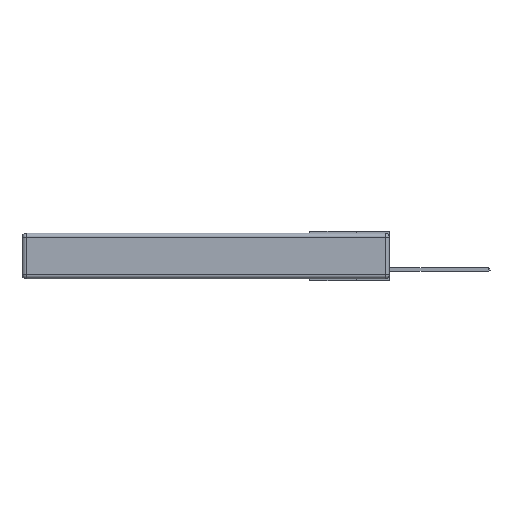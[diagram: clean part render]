
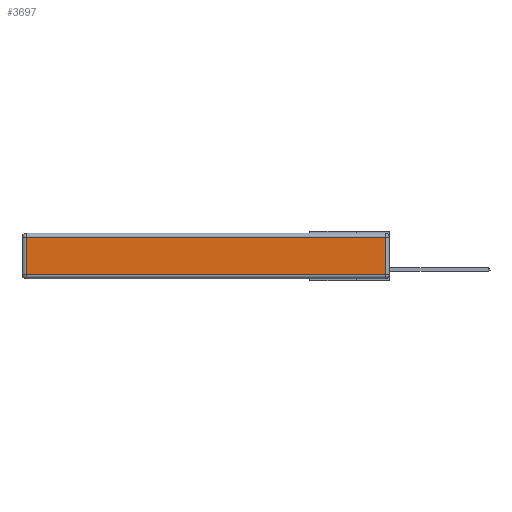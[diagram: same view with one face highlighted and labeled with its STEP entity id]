
A CAD part, left-side view. The second image highlights one B-rep face of the part: STEP entity #3697.
In plain terms, the highlighted planar face has unit normal (-1, 0, 0).
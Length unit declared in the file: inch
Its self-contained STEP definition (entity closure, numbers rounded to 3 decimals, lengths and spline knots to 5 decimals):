
#84 = VECTOR ( 'NONE', #12034, 39.37008 ) ;
#610 = PLANE ( 'NONE',  #6020 ) ;
#896 = VECTOR ( 'NONE', #3860, 39.37008 ) ;
#1994 = EDGE_LOOP ( 'NONE', ( #2185, #12031, #16019, #4994 ) ) ;
#2100 = CARTESIAN_POINT ( 'NONE',  ( 0., 0.03, -0.313 ) ) ;
#2173 = EDGE_CURVE ( 'NONE', #8842, #8181, #16119, .T. ) ;
#2185 = ORIENTED_EDGE ( 'NONE', *, *, #2173, .T. ) ;
#2301 = CARTESIAN_POINT ( 'NONE',  ( 0., 2.72, -0.03 ) ) ;
#2594 = CARTESIAN_POINT ( 'NONE',  ( 0., 0.03, -0.343 ) ) ;
#2646 = EDGE_CURVE ( 'NONE', #13889, #8842, #9479, .T. ) ;
#3697 = ADVANCED_FACE ( 'NONE', ( #5095 ), #610, .T. ) ;
#3860 = DIRECTION ( 'NONE',  ( 0., 0., 1. ) ) ;
#4325 = VERTEX_POINT ( 'NONE', #12150 ) ;
#4994 = ORIENTED_EDGE ( 'NONE', *, *, #2646, .T. ) ;
#5095 = FACE_OUTER_BOUND ( 'NONE', #1994, .T. ) ;
#6020 = AXIS2_PLACEMENT_3D ( 'NONE', #15780, #9581, #9794 ) ;
#6124 = VECTOR ( 'NONE', #11305, 39.37008 ) ;
#6652 = DIRECTION ( 'NONE',  ( 0., 1., 0. ) ) ;
#7256 = EDGE_CURVE ( 'NONE', #8181, #4325, #8352, .T. ) ;
#7280 = EDGE_CURVE ( 'NONE', #4325, #13889, #9692, .T. ) ;
#7716 = CARTESIAN_POINT ( 'NONE',  ( 0., 2.72, -0.313 ) ) ;
#8181 = VERTEX_POINT ( 'NONE', #2100 ) ;
#8352 = LINE ( 'NONE', #2594, #896 ) ;
#8842 = VERTEX_POINT ( 'NONE', #7716 ) ;
#9479 = LINE ( 'NONE', #14779, #6124 ) ;
#9581 = DIRECTION ( 'NONE',  ( -1., 0., 0. ) ) ;
#9692 = LINE ( 'NONE', #15462, #13408 ) ;
#9794 = DIRECTION ( 'NONE',  ( 0., 0., 1. ) ) ;
#11305 = DIRECTION ( 'NONE',  ( 0., 0., -1. ) ) ;
#11872 = CARTESIAN_POINT ( 'NONE',  ( 0., 0., -0.313 ) ) ;
#12031 = ORIENTED_EDGE ( 'NONE', *, *, #7256, .T. ) ;
#12034 = DIRECTION ( 'NONE',  ( 0., -1., 0. ) ) ;
#12150 = CARTESIAN_POINT ( 'NONE',  ( 0., 0.03, -0.03 ) ) ;
#13408 = VECTOR ( 'NONE', #6652, 39.37008 ) ;
#13889 = VERTEX_POINT ( 'NONE', #2301 ) ;
#14779 = CARTESIAN_POINT ( 'NONE',  ( 0., 2.72, -0.343 ) ) ;
#15462 = CARTESIAN_POINT ( 'NONE',  ( 0., 2.75, -0.03 ) ) ;
#15780 = CARTESIAN_POINT ( 'NONE',  ( 0., 0., -0.343 ) ) ;
#16019 = ORIENTED_EDGE ( 'NONE', *, *, #7280, .T. ) ;
#16119 = LINE ( 'NONE', #11872, #84 ) ;
